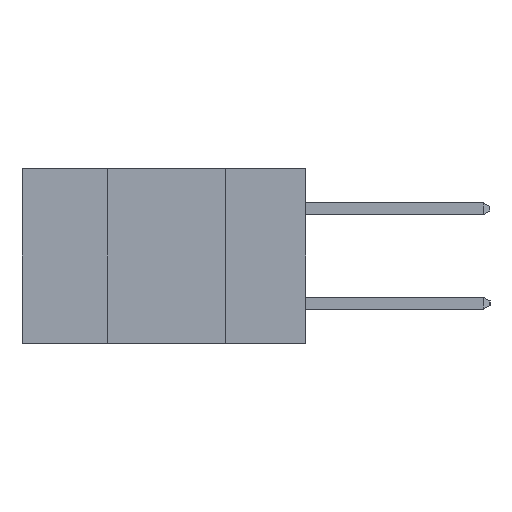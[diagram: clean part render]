
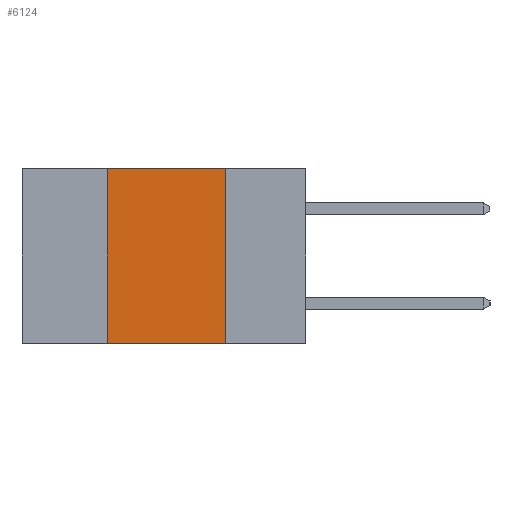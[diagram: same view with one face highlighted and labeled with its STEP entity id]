
A CAD part, left-side view. The second image highlights one B-rep face of the part: STEP entity #6124.
In plain terms, the highlighted planar face has unit normal (-1, 0, 0).
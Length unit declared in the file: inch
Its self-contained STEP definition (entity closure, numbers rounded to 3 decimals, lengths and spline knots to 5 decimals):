
#227 = VERTEX_POINT ( 'NONE', #15442 ) ;
#482 = DIRECTION ( 'NONE',  ( 0., 0., -1. ) ) ;
#504 = DIRECTION ( 'NONE',  ( 1., 0., 0. ) ) ;
#649 = CARTESIAN_POINT ( 'NONE',  ( 0., 0.6, 0. ) ) ;
#741 = EDGE_CURVE ( 'NONE', #227, #12890, #12072, .T. ) ;
#874 = PLANE ( 'NONE',  #17286 ) ;
#1586 = LINE ( 'NONE', #2312, #2056 ) ;
#1892 = CARTESIAN_POINT ( 'NONE',  ( 0., 0.17, -0.37 ) ) ;
#2056 = VECTOR ( 'NONE', #13739, 39.37008 ) ;
#2312 = CARTESIAN_POINT ( 'NONE',  ( 0., 0.6, -0.37 ) ) ;
#2768 = EDGE_CURVE ( 'NONE', #16340, #227, #13351, .T. ) ;
#3534 = CARTESIAN_POINT ( 'NONE',  ( 0., 0.6, 0. ) ) ;
#4500 = VECTOR ( 'NONE', #6109, 39.37008 ) ;
#5019 = ORIENTED_EDGE ( 'NONE', *, *, #2768, .F. ) ;
#5150 = CARTESIAN_POINT ( 'NONE',  ( 0., 0.42, 0. ) ) ;
#5378 = CARTESIAN_POINT ( 'NONE',  ( 0., 0.42, -0.37 ) ) ;
#5577 = DIRECTION ( 'NONE',  ( 0., 0., 1. ) ) ;
#5796 = VECTOR ( 'NONE', #6745, 39.37008 ) ;
#5816 = EDGE_CURVE ( 'NONE', #6346, #16340, #11232, .T. ) ;
#5912 = ORIENTED_EDGE ( 'NONE', *, *, #12381, .T. ) ;
#6109 = DIRECTION ( 'NONE',  ( 0., 0., -1. ) ) ;
#6124 = ADVANCED_FACE ( 'NONE', ( #10548 ), #874, .F. ) ;
#6246 = CARTESIAN_POINT ( 'NONE',  ( 0., 0.42, -0.37 ) ) ;
#6346 = VERTEX_POINT ( 'NONE', #6246 ) ;
#6745 = DIRECTION ( 'NONE',  ( 0., -1., 0. ) ) ;
#10548 = FACE_OUTER_BOUND ( 'NONE', #15855, .T. ) ;
#11232 = LINE ( 'NONE', #5378, #14991 ) ;
#12072 = LINE ( 'NONE', #16314, #4500 ) ;
#12381 = EDGE_CURVE ( 'NONE', #6346, #12890, #1586, .T. ) ;
#12890 = VERTEX_POINT ( 'NONE', #1892 ) ;
#13351 = LINE ( 'NONE', #3534, #5796 ) ;
#13739 = DIRECTION ( 'NONE',  ( 0., -1., 0. ) ) ;
#14991 = VECTOR ( 'NONE', #5577, 39.37008 ) ;
#15442 = CARTESIAN_POINT ( 'NONE',  ( 0., 0.17, 0. ) ) ;
#15848 = ORIENTED_EDGE ( 'NONE', *, *, #741, .F. ) ;
#15855 = EDGE_LOOP ( 'NONE', ( #15848, #5019, #16272, #5912 ) ) ;
#16272 = ORIENTED_EDGE ( 'NONE', *, *, #5816, .F. ) ;
#16314 = CARTESIAN_POINT ( 'NONE',  ( 0., 0.17, -0.37 ) ) ;
#16340 = VERTEX_POINT ( 'NONE', #5150 ) ;
#17286 = AXIS2_PLACEMENT_3D ( 'NONE', #649, #504, #482 ) ;
